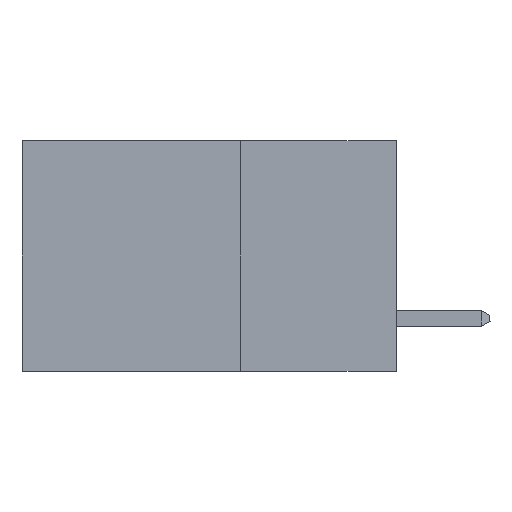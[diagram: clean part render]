
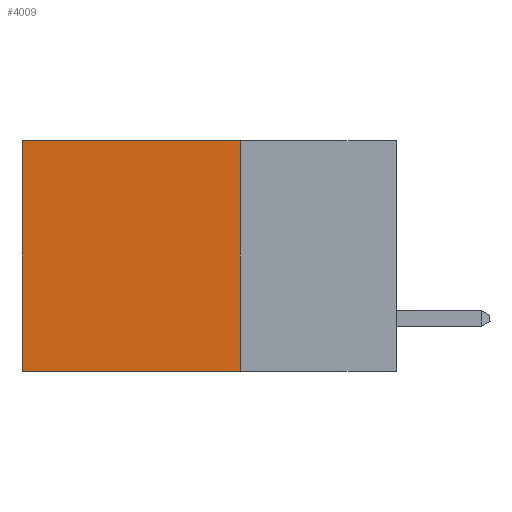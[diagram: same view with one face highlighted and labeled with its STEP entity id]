
A CAD part, left-side view. The second image highlights one B-rep face of the part: STEP entity #4009.
In plain terms, the highlighted planar face has unit normal (-1, 0, 0).
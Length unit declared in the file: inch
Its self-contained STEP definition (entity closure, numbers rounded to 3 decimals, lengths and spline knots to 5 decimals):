
#432 = VECTOR ( 'NONE', #13440, 39.37008 ) ;
#437 = ORIENTED_EDGE ( 'NONE', *, *, #6265, .T. ) ;
#736 = CARTESIAN_POINT ( 'NONE',  ( 0.298, 0.25, -0.37 ) ) ;
#796 = DIRECTION ( 'NONE',  ( 0., 0., -1. ) ) ;
#1566 = FACE_OUTER_BOUND ( 'NONE', #7293, .T. ) ;
#1867 = DIRECTION ( 'NONE',  ( 0., 1., 0. ) ) ;
#2271 = VECTOR ( 'NONE', #6191, 39.37008 ) ;
#2876 = VERTEX_POINT ( 'NONE', #4615 ) ;
#2881 = ORIENTED_EDGE ( 'NONE', *, *, #13069, .F. ) ;
#3102 = ORIENTED_EDGE ( 'NONE', *, *, #3941, .T. ) ;
#3454 = VERTEX_POINT ( 'NONE', #7375 ) ;
#3557 = CARTESIAN_POINT ( 'NONE',  ( 0.298, 0.25, 0. ) ) ;
#3677 = CARTESIAN_POINT ( 'NONE',  ( 0.298, 0.6, -0.37 ) ) ;
#3925 = DIRECTION ( 'NONE',  ( 1., 0., 0. ) ) ;
#3941 = EDGE_CURVE ( 'NONE', #2876, #7273, #5235, .T. ) ;
#4009 = ADVANCED_FACE ( 'NONE', ( #1566 ), #4905, .F. ) ;
#4109 = CARTESIAN_POINT ( 'NONE',  ( 0.298, 0.6, 0. ) ) ;
#4615 = CARTESIAN_POINT ( 'NONE',  ( 0.298, 0.6, 0. ) ) ;
#4905 = PLANE ( 'NONE',  #12483 ) ;
#5235 = LINE ( 'NONE', #4109, #2271 ) ;
#5667 = VECTOR ( 'NONE', #11018, 39.37008 ) ;
#6191 = DIRECTION ( 'NONE',  ( 0., 0., -1. ) ) ;
#6265 = EDGE_CURVE ( 'NONE', #11022, #2876, #13557, .T. ) ;
#6989 = CARTESIAN_POINT ( 'NONE',  ( 0.298, 0.25, 0. ) ) ;
#7273 = VERTEX_POINT ( 'NONE', #3677 ) ;
#7293 = EDGE_LOOP ( 'NONE', ( #3102, #2881, #7331, #437 ) ) ;
#7331 = ORIENTED_EDGE ( 'NONE', *, *, #7465, .F. ) ;
#7350 = CARTESIAN_POINT ( 'NONE',  ( 0.298, 0.25, 0. ) ) ;
#7375 = CARTESIAN_POINT ( 'NONE',  ( 0.298, 0.25, -0.37 ) ) ;
#7465 = EDGE_CURVE ( 'NONE', #11022, #3454, #9225, .T. ) ;
#9225 = LINE ( 'NONE', #13426, #432 ) ;
#9768 = VECTOR ( 'NONE', #1867, 39.37008 ) ;
#11018 = DIRECTION ( 'NONE',  ( 0., 1., 0. ) ) ;
#11022 = VERTEX_POINT ( 'NONE', #6989 ) ;
#12483 = AXIS2_PLACEMENT_3D ( 'NONE', #3557, #3925, #796 ) ;
#12577 = LINE ( 'NONE', #736, #9768 ) ;
#13069 = EDGE_CURVE ( 'NONE', #3454, #7273, #12577, .T. ) ;
#13426 = CARTESIAN_POINT ( 'NONE',  ( 0.298, 0.25, 0. ) ) ;
#13440 = DIRECTION ( 'NONE',  ( 0., 0., -1. ) ) ;
#13557 = LINE ( 'NONE', #7350, #5667 ) ;
